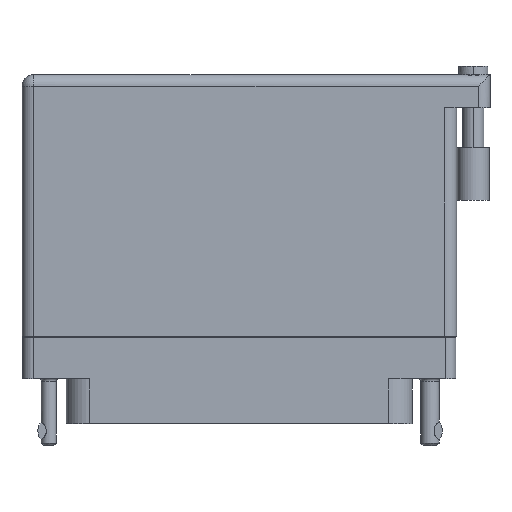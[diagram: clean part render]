
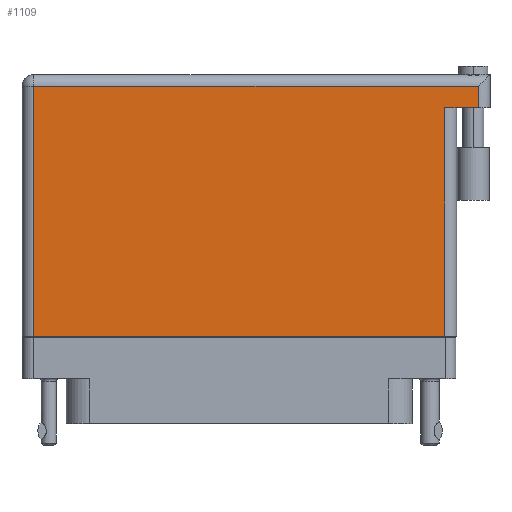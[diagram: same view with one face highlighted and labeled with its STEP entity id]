
A CAD part, front view. The second image highlights one B-rep face of the part: STEP entity #1109.
In plain terms, the highlighted face is planar.
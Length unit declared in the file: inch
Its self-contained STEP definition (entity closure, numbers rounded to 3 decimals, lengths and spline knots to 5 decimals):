
#646 = CARTESIAN_POINT ( 'NONE',  ( 1.43, 1.269, 0.4495 ) ) ;
#892 = DIRECTION ( 'NONE',  ( -1., 0., 0. ) ) ;
#967 = EDGE_CURVE ( 'NONE', #12461, #53837, #52766, .T. ) ;
#1109 = ADVANCED_FACE ( 'NONE', ( #29235 ), #38874, .F. ) ;
#2050 = EDGE_CURVE ( 'NONE', #53837, #19466, #9398, .T. ) ;
#2437 = DIRECTION ( 'NONE',  ( -1., 0., 0. ) ) ;
#4620 = EDGE_CURVE ( 'NONE', #50531, #19466, #30099, .T. ) ;
#4686 = LINE ( 'NONE', #39436, #19445 ) ;
#6487 = CARTESIAN_POINT ( 'NONE',  ( 1.23, 1.269, 0.4495 ) ) ;
#6758 = VERTEX_POINT ( 'NONE', #51740 ) ;
#9398 = LINE ( 'NONE', #6487, #56397 ) ;
#10858 = AXIS2_PLACEMENT_3D ( 'NONE', #38268, #24487, #892 ) ;
#12398 = EDGE_CURVE ( 'NONE', #6758, #12461, #57190, .T. ) ;
#12461 = VERTEX_POINT ( 'NONE', #15423 ) ;
#12488 = VECTOR ( 'NONE', #2437, 39.37008 ) ;
#15423 = CARTESIAN_POINT ( 'NONE',  ( -1.23, -0.1, 0.4495 ) ) ;
#15837 = DIRECTION ( 'NONE',  ( 0., 1., 0. ) ) ;
#16945 = CARTESIAN_POINT ( 'NONE',  ( -1.3, 1.396, 0.4495 ) ) ;
#18537 = EDGE_LOOP ( 'NONE', ( #26749, #27732, #20600, #35409, #25873, #36806 ) ) ;
#18710 = CARTESIAN_POINT ( 'NONE',  ( 1.23, 1.269, 0.4495 ) ) ;
#19445 = VECTOR ( 'NONE', #15837, 39.37008 ) ;
#19466 = VERTEX_POINT ( 'NONE', #18710 ) ;
#20600 = ORIENTED_EDGE ( 'NONE', *, *, #4620, .F. ) ;
#21326 = CARTESIAN_POINT ( 'NONE',  ( 1.5, 1.269, 0.4495 ) ) ;
#24487 = DIRECTION ( 'NONE',  ( 0., 0., -1. ) ) ;
#25873 = ORIENTED_EDGE ( 'NONE', *, *, #46633, .T. ) ;
#26749 = ORIENTED_EDGE ( 'NONE', *, *, #967, .T. ) ;
#27732 = ORIENTED_EDGE ( 'NONE', *, *, #2050, .T. ) ;
#29235 = FACE_OUTER_BOUND ( 'NONE', #18537, .T. ) ;
#30099 = LINE ( 'NONE', #21326, #12488 ) ;
#32274 = DIRECTION ( 'NONE',  ( -1., 0., 0. ) ) ;
#32685 = VERTEX_POINT ( 'NONE', #39988 ) ;
#33231 = CARTESIAN_POINT ( 'NONE',  ( -1.23, -0.1, 0.4495 ) ) ;
#34924 = CARTESIAN_POINT ( 'NONE',  ( 1.23, -0.1, 0.4495 ) ) ;
#35409 = ORIENTED_EDGE ( 'NONE', *, *, #54753, .T. ) ;
#36806 = ORIENTED_EDGE ( 'NONE', *, *, #12398, .T. ) ;
#37048 = CARTESIAN_POINT ( 'NONE',  ( -1.3, -0.1, 0.4495 ) ) ;
#38268 = CARTESIAN_POINT ( 'NONE',  ( -1.3, 1.466, 0.4495 ) ) ;
#38874 = PLANE ( 'NONE',  #10858 ) ;
#39436 = CARTESIAN_POINT ( 'NONE',  ( 1.43, 1.466, 0.4495 ) ) ;
#39988 = CARTESIAN_POINT ( 'NONE',  ( 1.43, 1.396, 0.4495 ) ) ;
#43274 = VECTOR ( 'NONE', #55795, 39.37008 ) ;
#46633 = EDGE_CURVE ( 'NONE', #32685, #6758, #47318, .T. ) ;
#47318 = LINE ( 'NONE', #16945, #58252 ) ;
#50531 = VERTEX_POINT ( 'NONE', #646 ) ;
#50563 = VECTOR ( 'NONE', #60387, 39.37008 ) ;
#51740 = CARTESIAN_POINT ( 'NONE',  ( -1.23, 1.396, 0.4495 ) ) ;
#52668 = DIRECTION ( 'NONE',  ( 0., 1., 0. ) ) ;
#52766 = LINE ( 'NONE', #37048, #50563 ) ;
#53837 = VERTEX_POINT ( 'NONE', #34924 ) ;
#54753 = EDGE_CURVE ( 'NONE', #50531, #32685, #4686, .T. ) ;
#55795 = DIRECTION ( 'NONE',  ( 0., -1., 0. ) ) ;
#56397 = VECTOR ( 'NONE', #52668, 39.37008 ) ;
#57190 = LINE ( 'NONE', #33231, #43274 ) ;
#58252 = VECTOR ( 'NONE', #32274, 39.37008 ) ;
#60387 = DIRECTION ( 'NONE',  ( 1., 0., 0. ) ) ;
